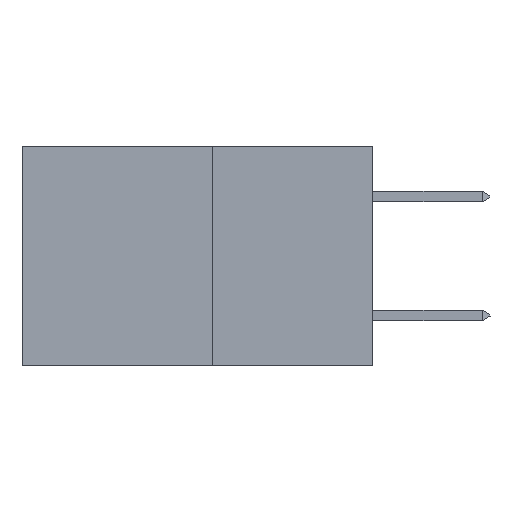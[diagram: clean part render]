
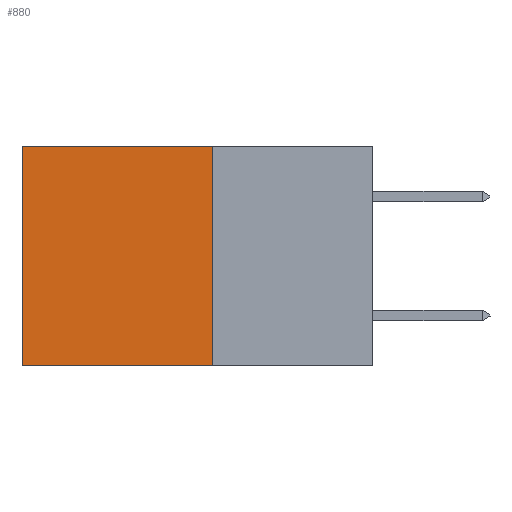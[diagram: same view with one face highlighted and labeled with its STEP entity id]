
A CAD part, left-side view. The second image highlights one B-rep face of the part: STEP entity #880.
In plain terms, the highlighted planar face has unit normal (-1, 0, 0).
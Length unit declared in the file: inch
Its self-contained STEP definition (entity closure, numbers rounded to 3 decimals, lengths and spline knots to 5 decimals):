
#165 = LINE ( 'NONE', #5178, #2461 ) ;
#375 = VERTEX_POINT ( 'NONE', #4082 ) ;
#672 = CARTESIAN_POINT ( 'NONE',  ( 0.277, 0.27, 0. ) ) ;
#690 = DIRECTION ( 'NONE',  ( 0., 1., 0. ) ) ;
#880 = ADVANCED_FACE ( 'NONE', ( #8681 ), #4660, .F. ) ;
#2088 = VECTOR ( 'NONE', #6577, 39.37008 ) ;
#2195 = VERTEX_POINT ( 'NONE', #5929 ) ;
#2461 = VECTOR ( 'NONE', #2690, 39.37008 ) ;
#2482 = DIRECTION ( 'NONE',  ( 1., 0., 0. ) ) ;
#2493 = CARTESIAN_POINT ( 'NONE',  ( 0.277, 0.59, -0.37 ) ) ;
#2690 = DIRECTION ( 'NONE',  ( 0., 1., 0. ) ) ;
#2946 = DIRECTION ( 'NONE',  ( 0., 0., -1. ) ) ;
#3239 = VERTEX_POINT ( 'NONE', #8318 ) ;
#3263 = EDGE_CURVE ( 'NONE', #3546, #375, #5241, .T. ) ;
#3546 = VERTEX_POINT ( 'NONE', #7424 ) ;
#4082 = CARTESIAN_POINT ( 'NONE',  ( 0.277, 0.27, -0.37 ) ) ;
#4466 = VECTOR ( 'NONE', #9052, 39.37008 ) ;
#4660 = PLANE ( 'NONE',  #5733 ) ;
#4675 = CARTESIAN_POINT ( 'NONE',  ( 0.277, 0.27, -0.37 ) ) ;
#5178 = CARTESIAN_POINT ( 'NONE',  ( 0.277, 0.27, -0.37 ) ) ;
#5241 = LINE ( 'NONE', #9029, #4466 ) ;
#5416 = EDGE_LOOP ( 'NONE', ( #7011, #7489, #5879, #6373 ) ) ;
#5733 = AXIS2_PLACEMENT_3D ( 'NONE', #4675, #2482, #2946 ) ;
#5879 = ORIENTED_EDGE ( 'NONE', *, *, #3263, .F. ) ;
#5929 = CARTESIAN_POINT ( 'NONE',  ( 0.277, 0.59, 0. ) ) ;
#5945 = EDGE_CURVE ( 'NONE', #3546, #2195, #8442, .T. ) ;
#6366 = VECTOR ( 'NONE', #690, 39.37008 ) ;
#6373 = ORIENTED_EDGE ( 'NONE', *, *, #5945, .T. ) ;
#6577 = DIRECTION ( 'NONE',  ( 0., 0., -1. ) ) ;
#6727 = EDGE_CURVE ( 'NONE', #2195, #3239, #10212, .T. ) ;
#7011 = ORIENTED_EDGE ( 'NONE', *, *, #6727, .T. ) ;
#7424 = CARTESIAN_POINT ( 'NONE',  ( 0.277, 0.27, 0. ) ) ;
#7489 = ORIENTED_EDGE ( 'NONE', *, *, #8349, .F. ) ;
#8318 = CARTESIAN_POINT ( 'NONE',  ( 0.277, 0.59, -0.37 ) ) ;
#8349 = EDGE_CURVE ( 'NONE', #375, #3239, #165, .T. ) ;
#8442 = LINE ( 'NONE', #672, #6366 ) ;
#8681 = FACE_OUTER_BOUND ( 'NONE', #5416, .T. ) ;
#9029 = CARTESIAN_POINT ( 'NONE',  ( 0.277, 0.27, -0.37 ) ) ;
#9052 = DIRECTION ( 'NONE',  ( 0., 0., -1. ) ) ;
#10212 = LINE ( 'NONE', #2493, #2088 ) ;
